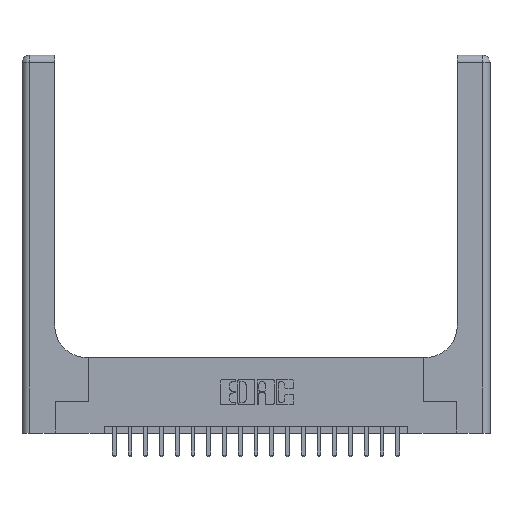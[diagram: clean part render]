
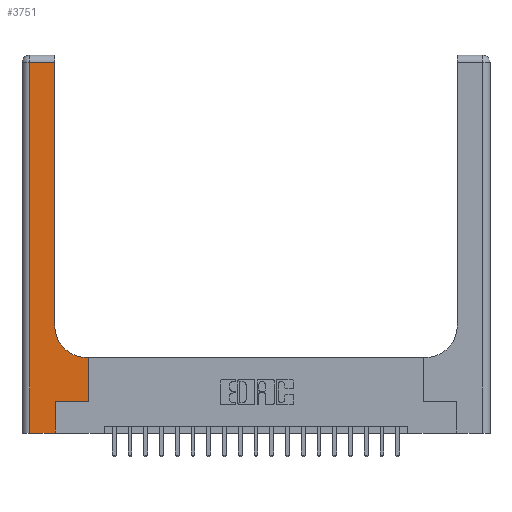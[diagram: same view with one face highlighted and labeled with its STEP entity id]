
A CAD part, top view. The second image highlights one B-rep face of the part: STEP entity #3751.
In plain terms, the highlighted planar face has unit normal (0, 0, 1).
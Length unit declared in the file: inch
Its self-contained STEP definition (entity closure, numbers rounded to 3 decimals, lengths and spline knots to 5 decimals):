
#582 = CARTESIAN_POINT ( 'NONE',  ( 0.06, 0., 0.37 ) ) ;
#758 = EDGE_CURVE ( 'NONE', #16480, #6381, #18811, .T. ) ;
#825 = EDGE_CURVE ( 'NONE', #17081, #16480, #7197, .T. ) ;
#830 = ORIENTED_EDGE ( 'NONE', *, *, #3997, .T. ) ;
#981 = ORIENTED_EDGE ( 'NONE', *, *, #1076, .T. ) ;
#1076 = EDGE_CURVE ( 'NONE', #16852, #17459, #5588, .T. ) ;
#1151 = VECTOR ( 'NONE', #19961, 39.37008 ) ;
#1459 = ORIENTED_EDGE ( 'NONE', *, *, #11159, .T. ) ;
#1679 = EDGE_CURVE ( 'NONE', #17846, #17081, #5089, .T. ) ;
#1763 = CARTESIAN_POINT ( 'NONE',  ( 0.51, 0.6, 0.37 ) ) ;
#2127 = VECTOR ( 'NONE', #4159, 39.37008 ) ;
#2416 = LINE ( 'NONE', #10474, #4715 ) ;
#2571 = DIRECTION ( 'NONE',  ( 1., 0., 0. ) ) ;
#3311 = EDGE_CURVE ( 'NONE', #17574, #9354, #15519, .T. ) ;
#3423 = CARTESIAN_POINT ( 'NONE',  ( 0.265, 0., 0.37 ) ) ;
#3751 = ADVANCED_FACE ( 'NONE', ( #13862 ), #5687, .F. ) ;
#3878 = CARTESIAN_POINT ( 'NONE',  ( 0., 0., 0.37 ) ) ;
#3942 = AXIS2_PLACEMENT_3D ( 'NONE', #16870, #13546, #5369 ) ;
#3997 = EDGE_CURVE ( 'NONE', #15158, #16852, #10065, .T. ) ;
#4159 = DIRECTION ( 'NONE',  ( 0., 1., 0. ) ) ;
#4666 = DIRECTION ( 'NONE',  ( -1., 0., 0. ) ) ;
#4715 = VECTOR ( 'NONE', #18857, 39.37008 ) ;
#5089 = LINE ( 'NONE', #11322, #5161 ) ;
#5134 = ORIENTED_EDGE ( 'NONE', *, *, #758, .T. ) ;
#5161 = VECTOR ( 'NONE', #4666, 39.37008 ) ;
#5302 = DIRECTION ( 'NONE',  ( 0., -1., 0. ) ) ;
#5369 = DIRECTION ( 'NONE',  ( -1., 0., 0. ) ) ;
#5588 = LINE ( 'NONE', #9404, #14418 ) ;
#5687 = PLANE ( 'NONE',  #3942 ) ;
#6381 = VERTEX_POINT ( 'NONE', #10654 ) ;
#6674 = EDGE_CURVE ( 'NONE', #17459, #17846, #14948, .T. ) ;
#7154 = CARTESIAN_POINT ( 'NONE',  ( 0.528, 0.6, 0.37 ) ) ;
#7197 = CIRCLE ( 'NONE', #18498, 0.25 ) ;
#7737 = DIRECTION ( 'NONE',  ( 0., 0., -1. ) ) ;
#8222 = ORIENTED_EDGE ( 'NONE', *, *, #825, .T. ) ;
#8666 = ORIENTED_EDGE ( 'NONE', *, *, #1679, .T. ) ;
#9354 = VERTEX_POINT ( 'NONE', #582 ) ;
#9404 = CARTESIAN_POINT ( 'NONE',  ( 0.265, 0.25, 0.37 ) ) ;
#10065 = LINE ( 'NONE', #3423, #1151 ) ;
#10474 = CARTESIAN_POINT ( 'NONE',  ( 0., 2.94, 0.37 ) ) ;
#10654 = CARTESIAN_POINT ( 'NONE',  ( 0.26, 2.94, 0.37 ) ) ;
#10655 = CARTESIAN_POINT ( 'NONE',  ( 0.26, 3., 0.37 ) ) ;
#10950 = ORIENTED_EDGE ( 'NONE', *, *, #3311, .T. ) ;
#11159 = EDGE_CURVE ( 'NONE', #9354, #15158, #15385, .T. ) ;
#11322 = CARTESIAN_POINT ( 'NONE',  ( 0.26, 0.6, 0.37 ) ) ;
#11501 = CARTESIAN_POINT ( 'NONE',  ( 0.51, 0.85, 0.37 ) ) ;
#12032 = ORIENTED_EDGE ( 'NONE', *, *, #6674, .T. ) ;
#12155 = CARTESIAN_POINT ( 'NONE',  ( 0.06, 2.94, 0.37 ) ) ;
#13390 = VECTOR ( 'NONE', #17218, 39.37008 ) ;
#13546 = DIRECTION ( 'NONE',  ( 0., 0., -1. ) ) ;
#13862 = FACE_OUTER_BOUND ( 'NONE', #14986, .T. ) ;
#13898 = CARTESIAN_POINT ( 'NONE',  ( 0.06, 3., 0.37 ) ) ;
#14418 = VECTOR ( 'NONE', #17584, 39.37008 ) ;
#14948 = LINE ( 'NONE', #18875, #2127 ) ;
#14986 = EDGE_LOOP ( 'NONE', ( #5134, #18394, #10950, #1459, #830, #981, #12032, #8666, #8222 ) ) ;
#15158 = VERTEX_POINT ( 'NONE', #18204 ) ;
#15172 = CARTESIAN_POINT ( 'NONE',  ( 0.528, 0.25, 0.37 ) ) ;
#15385 = LINE ( 'NONE', #3878, #19221 ) ;
#15519 = LINE ( 'NONE', #13898, #20117 ) ;
#16179 = CARTESIAN_POINT ( 'NONE',  ( 0.265, 0.25, 0.37 ) ) ;
#16480 = VERTEX_POINT ( 'NONE', #19192 ) ;
#16732 = EDGE_CURVE ( 'NONE', #6381, #17574, #2416, .T. ) ;
#16852 = VERTEX_POINT ( 'NONE', #16179 ) ;
#16870 = CARTESIAN_POINT ( 'NONE',  ( 0., 3., 0.37 ) ) ;
#17081 = VERTEX_POINT ( 'NONE', #1763 ) ;
#17218 = DIRECTION ( 'NONE',  ( 0., 1., 0. ) ) ;
#17459 = VERTEX_POINT ( 'NONE', #15172 ) ;
#17574 = VERTEX_POINT ( 'NONE', #12155 ) ;
#17584 = DIRECTION ( 'NONE',  ( 1., 0., 0. ) ) ;
#17631 = DIRECTION ( 'NONE',  ( 1., 0., 0. ) ) ;
#17846 = VERTEX_POINT ( 'NONE', #7154 ) ;
#18204 = CARTESIAN_POINT ( 'NONE',  ( 0.265, 0., 0.37 ) ) ;
#18394 = ORIENTED_EDGE ( 'NONE', *, *, #16732, .T. ) ;
#18498 = AXIS2_PLACEMENT_3D ( 'NONE', #11501, #7737, #17631 ) ;
#18811 = LINE ( 'NONE', #10655, #13390 ) ;
#18857 = DIRECTION ( 'NONE',  ( -1., 0., 0. ) ) ;
#18875 = CARTESIAN_POINT ( 'NONE',  ( 0.528, 0.25, 0.37 ) ) ;
#19192 = CARTESIAN_POINT ( 'NONE',  ( 0.26, 0.85, 0.37 ) ) ;
#19221 = VECTOR ( 'NONE', #2571, 39.37008 ) ;
#19961 = DIRECTION ( 'NONE',  ( 0., 1., 0. ) ) ;
#20117 = VECTOR ( 'NONE', #5302, 39.37008 ) ;
